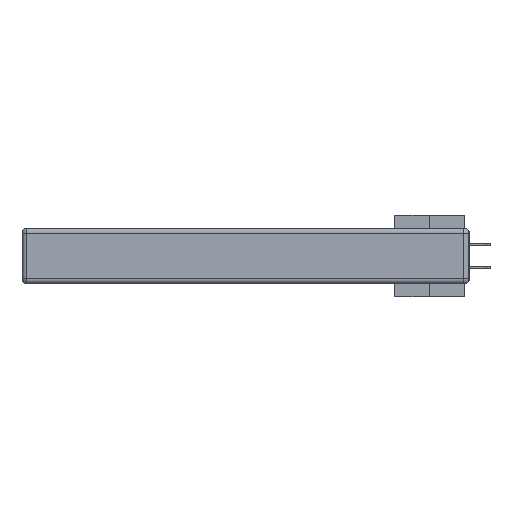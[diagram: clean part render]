
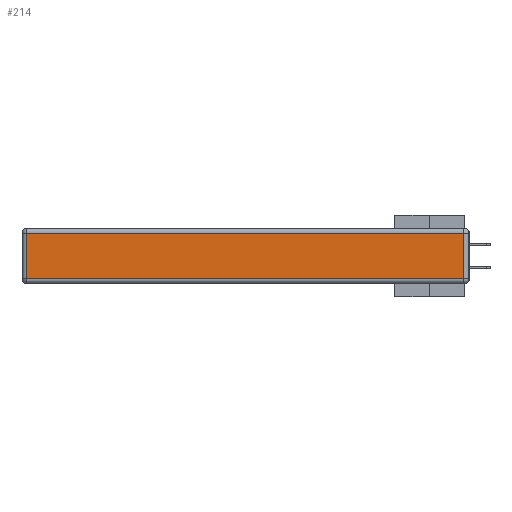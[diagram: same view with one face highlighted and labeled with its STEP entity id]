
A CAD part, left-side view. The second image highlights one B-rep face of the part: STEP entity #214.
In plain terms, the highlighted planar face has unit normal (-1, 0, 0).
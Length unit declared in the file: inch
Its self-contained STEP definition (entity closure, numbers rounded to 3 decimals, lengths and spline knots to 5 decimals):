
#214 = ADVANCED_FACE ( 'NONE', ( #20109 ), #31934, .T. ) ;
#311 = CARTESIAN_POINT ( 'NONE',  ( 0., 0.03, -0.313 ) ) ;
#2274 = CARTESIAN_POINT ( 'NONE',  ( 0., 0.03, -0.343 ) ) ;
#4003 = CARTESIAN_POINT ( 'NONE',  ( 0., 0., -0.313 ) ) ;
#5525 = LINE ( 'NONE', #2274, #20307 ) ;
#6076 = LINE ( 'NONE', #27496, #36102 ) ;
#6325 = EDGE_CURVE ( 'NONE', #9796, #16901, #5525, .T. ) ;
#7914 = ORIENTED_EDGE ( 'NONE', *, *, #10398, .T. ) ;
#9016 = ORIENTED_EDGE ( 'NONE', *, *, #6325, .T. ) ;
#9671 = DIRECTION ( 'NONE',  ( 0., 1., 0. ) ) ;
#9796 = VERTEX_POINT ( 'NONE', #311 ) ;
#10398 = EDGE_CURVE ( 'NONE', #16901, #20092, #6076, .T. ) ;
#10763 = CARTESIAN_POINT ( 'NONE',  ( 0., 0., -0.343 ) ) ;
#16468 = CARTESIAN_POINT ( 'NONE',  ( 0., 0.03, -0.03 ) ) ;
#16786 = VECTOR ( 'NONE', #25313, 39.37008 ) ;
#16901 = VERTEX_POINT ( 'NONE', #16468 ) ;
#17291 = ORIENTED_EDGE ( 'NONE', *, *, #23923, .T. ) ;
#17732 = LINE ( 'NONE', #4003, #16786 ) ;
#20092 = VERTEX_POINT ( 'NONE', #36453 ) ;
#20109 = FACE_OUTER_BOUND ( 'NONE', #23297, .T. ) ;
#20307 = VECTOR ( 'NONE', #35985, 39.37008 ) ;
#21888 = EDGE_CURVE ( 'NONE', #38157, #9796, #17732, .T. ) ;
#21965 = ORIENTED_EDGE ( 'NONE', *, *, #21888, .T. ) ;
#22885 = LINE ( 'NONE', #38009, #36636 ) ;
#23297 = EDGE_LOOP ( 'NONE', ( #21965, #9016, #7914, #17291 ) ) ;
#23923 = EDGE_CURVE ( 'NONE', #20092, #38157, #22885, .T. ) ;
#25313 = DIRECTION ( 'NONE',  ( 0., -1., 0. ) ) ;
#27496 = CARTESIAN_POINT ( 'NONE',  ( 0., 2.75, -0.03 ) ) ;
#29219 = DIRECTION ( 'NONE',  ( 0., 0., -1. ) ) ;
#30357 = AXIS2_PLACEMENT_3D ( 'NONE', #10763, #32059, #35140 ) ;
#31052 = CARTESIAN_POINT ( 'NONE',  ( 0., 2.72, -0.313 ) ) ;
#31934 = PLANE ( 'NONE',  #30357 ) ;
#32059 = DIRECTION ( 'NONE',  ( -1., 0., 0. ) ) ;
#35140 = DIRECTION ( 'NONE',  ( 0., 0., 1. ) ) ;
#35985 = DIRECTION ( 'NONE',  ( 0., 0., 1. ) ) ;
#36102 = VECTOR ( 'NONE', #9671, 39.37008 ) ;
#36453 = CARTESIAN_POINT ( 'NONE',  ( 0., 2.72, -0.03 ) ) ;
#36636 = VECTOR ( 'NONE', #29219, 39.37008 ) ;
#38009 = CARTESIAN_POINT ( 'NONE',  ( 0., 2.72, -0.343 ) ) ;
#38157 = VERTEX_POINT ( 'NONE', #31052 ) ;
